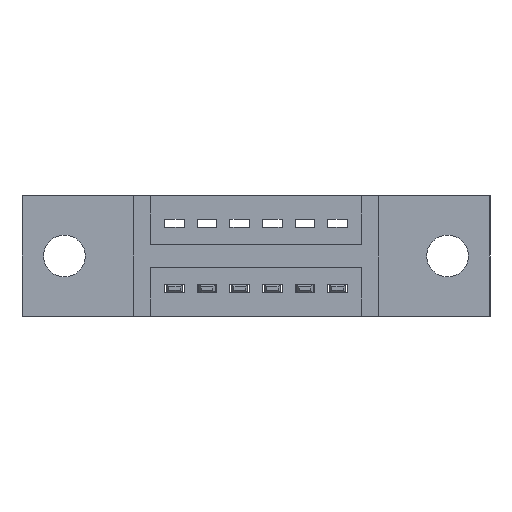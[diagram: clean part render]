
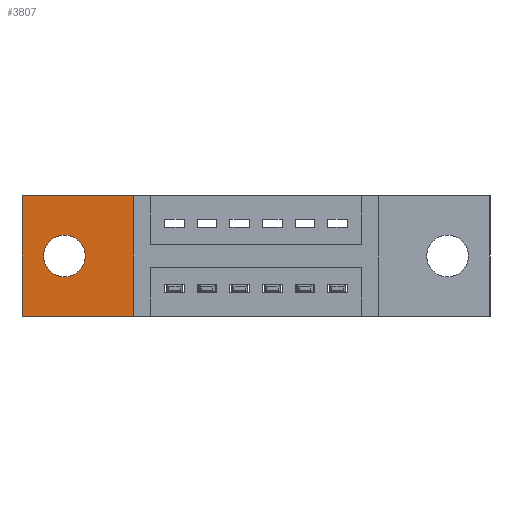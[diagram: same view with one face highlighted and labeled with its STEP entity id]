
A CAD part, front view. The second image highlights one B-rep face of the part: STEP entity #3807.
In plain terms, the highlighted planar face has unit normal (0, -1, 0).
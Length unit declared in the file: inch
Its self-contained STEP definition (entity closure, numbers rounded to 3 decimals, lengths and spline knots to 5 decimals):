
#96 = DIRECTION ( 'NONE',  ( 0., 0., -1. ) ) ;
#183 = FACE_BOUND ( 'NONE', #8770, .T. ) ;
#202 = CARTESIAN_POINT ( 'NONE',  ( 0., 0.11, -0.37 ) ) ;
#247 = AXIS2_PLACEMENT_3D ( 'NONE', #4222, #7386, #7673 ) ;
#674 = VERTEX_POINT ( 'NONE', #8879 ) ;
#705 = ORIENTED_EDGE ( 'NONE', *, *, #4711, .F. ) ;
#955 = ORIENTED_EDGE ( 'NONE', *, *, #3764, .T. ) ;
#971 = VECTOR ( 'NONE', #2657, 39.37008 ) ;
#1025 = CARTESIAN_POINT ( 'NONE',  ( 0.13, 0.11, -0.185 ) ) ;
#1026 = DIRECTION ( 'NONE',  ( 0., -1., 0. ) ) ;
#1069 = DIRECTION ( 'NONE',  ( 0., 0., -1. ) ) ;
#1308 = VERTEX_POINT ( 'NONE', #3585 ) ;
#1418 = VERTEX_POINT ( 'NONE', #2131 ) ;
#1685 = EDGE_CURVE ( 'NONE', #2201, #2154, #4563, .T. ) ;
#1854 = CARTESIAN_POINT ( 'NONE',  ( 0., 0.11, 0. ) ) ;
#1981 = CARTESIAN_POINT ( 'NONE',  ( 0., 0.11, 0. ) ) ;
#2131 = CARTESIAN_POINT ( 'NONE',  ( 0.13, 0.11, -0.121 ) ) ;
#2154 = VERTEX_POINT ( 'NONE', #202 ) ;
#2173 = CIRCLE ( 'NONE', #5251, 0.064 ) ;
#2201 = VERTEX_POINT ( 'NONE', #1854 ) ;
#2340 = CARTESIAN_POINT ( 'NONE',  ( 0., 0.11, -0.37 ) ) ;
#2640 = CARTESIAN_POINT ( 'NONE',  ( 0.3425, 0.11, 0. ) ) ;
#2657 = DIRECTION ( 'NONE',  ( 0., 0., 1. ) ) ;
#2727 = CIRCLE ( 'NONE', #247, 0.064 ) ;
#2952 = ORIENTED_EDGE ( 'NONE', *, *, #1685, .T. ) ;
#2968 = LINE ( 'NONE', #2640, #971 ) ;
#3106 = EDGE_CURVE ( 'NONE', #2154, #674, #6799, .T. ) ;
#3112 = VECTOR ( 'NONE', #5386, 39.37008 ) ;
#3206 = ORIENTED_EDGE ( 'NONE', *, *, #8191, .T. ) ;
#3356 = EDGE_CURVE ( 'NONE', #5266, #1418, #2727, .T. ) ;
#3585 = CARTESIAN_POINT ( 'NONE',  ( 0.3425, 0.11, 0. ) ) ;
#3632 = DIRECTION ( 'NONE',  ( 0., -1., 0. ) ) ;
#3655 = DIRECTION ( 'NONE',  ( 0., 0., -1. ) ) ;
#3764 = EDGE_CURVE ( 'NONE', #674, #1308, #2968, .T. ) ;
#3807 = ADVANCED_FACE ( 'NONE', ( #183, #7581 ), #7146, .T. ) ;
#4222 = CARTESIAN_POINT ( 'NONE',  ( 0.13, 0.11, -0.185 ) ) ;
#4563 = LINE ( 'NONE', #8730, #6016 ) ;
#4711 = EDGE_CURVE ( 'NONE', #1418, #5266, #2173, .T. ) ;
#4846 = ORIENTED_EDGE ( 'NONE', *, *, #3356, .F. ) ;
#5251 = AXIS2_PLACEMENT_3D ( 'NONE', #1025, #1026, #1069 ) ;
#5266 = VERTEX_POINT ( 'NONE', #8255 ) ;
#5386 = DIRECTION ( 'NONE',  ( 1., 0., 0. ) ) ;
#5409 = EDGE_LOOP ( 'NONE', ( #2952, #8391, #955, #3206 ) ) ;
#6016 = VECTOR ( 'NONE', #96, 39.37008 ) ;
#6731 = CARTESIAN_POINT ( 'NONE',  ( 0., 0.11, -0.37 ) ) ;
#6799 = LINE ( 'NONE', #2340, #3112 ) ;
#6977 = LINE ( 'NONE', #1981, #8884 ) ;
#7146 = PLANE ( 'NONE',  #7496 ) ;
#7386 = DIRECTION ( 'NONE',  ( 0., -1., 0. ) ) ;
#7496 = AXIS2_PLACEMENT_3D ( 'NONE', #6731, #3632, #3655 ) ;
#7581 = FACE_OUTER_BOUND ( 'NONE', #5409, .T. ) ;
#7673 = DIRECTION ( 'NONE',  ( 0., 0., -1. ) ) ;
#8191 = EDGE_CURVE ( 'NONE', #1308, #2201, #6977, .T. ) ;
#8255 = CARTESIAN_POINT ( 'NONE',  ( 0.13, 0.11, -0.249 ) ) ;
#8311 = DIRECTION ( 'NONE',  ( -1., 0., 0. ) ) ;
#8391 = ORIENTED_EDGE ( 'NONE', *, *, #3106, .T. ) ;
#8730 = CARTESIAN_POINT ( 'NONE',  ( 0., 0.11, 0. ) ) ;
#8770 = EDGE_LOOP ( 'NONE', ( #705, #4846 ) ) ;
#8879 = CARTESIAN_POINT ( 'NONE',  ( 0.3425, 0.11, -0.37 ) ) ;
#8884 = VECTOR ( 'NONE', #8311, 39.37008 ) ;
